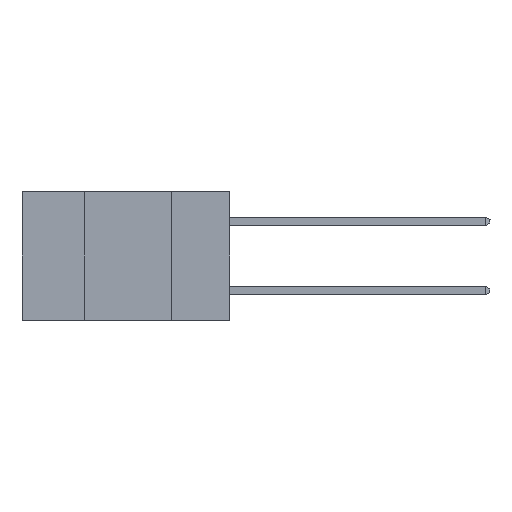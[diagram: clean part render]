
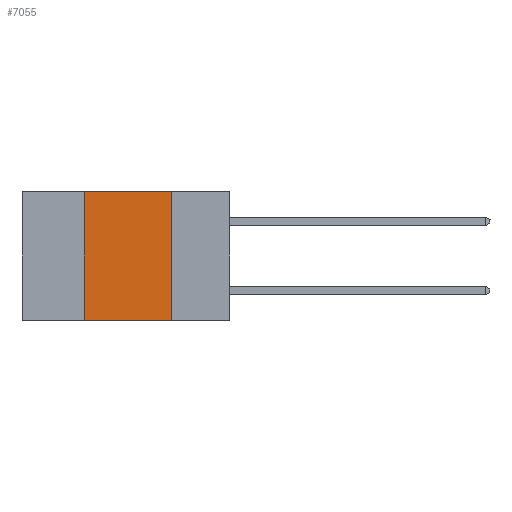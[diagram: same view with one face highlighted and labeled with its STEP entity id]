
A CAD part, left-side view. The second image highlights one B-rep face of the part: STEP entity #7055.
In plain terms, the highlighted planar face has unit normal (-1, 0, 0).
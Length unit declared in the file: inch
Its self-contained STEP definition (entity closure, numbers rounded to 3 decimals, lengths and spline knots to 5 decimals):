
#540 = CARTESIAN_POINT ( 'NONE',  ( 0., 0.6, 0. ) ) ;
#1301 = VECTOR ( 'NONE', #3598, 39.37008 ) ;
#1586 = PLANE ( 'NONE',  #12583 ) ;
#1851 = EDGE_CURVE ( 'NONE', #7175, #4933, #13333, .T. ) ;
#2065 = VECTOR ( 'NONE', #4956, 39.37008 ) ;
#2358 = EDGE_CURVE ( 'NONE', #7175, #4273, #6898, .T. ) ;
#2370 = EDGE_LOOP ( 'NONE', ( #14096, #10110, #2570, #3733 ) ) ;
#2570 = ORIENTED_EDGE ( 'NONE', *, *, #1851, .F. ) ;
#2785 = DIRECTION ( 'NONE',  ( 1., 0., 0. ) ) ;
#3254 = DIRECTION ( 'NONE',  ( 0., 0., 1. ) ) ;
#3525 = CARTESIAN_POINT ( 'NONE',  ( 0., 0.17, -0.37 ) ) ;
#3598 = DIRECTION ( 'NONE',  ( 0., 0., -1. ) ) ;
#3733 = ORIENTED_EDGE ( 'NONE', *, *, #2358, .T. ) ;
#4273 = VERTEX_POINT ( 'NONE', #9576 ) ;
#4481 = VECTOR ( 'NONE', #11503, 39.37008 ) ;
#4933 = VERTEX_POINT ( 'NONE', #9514 ) ;
#4956 = DIRECTION ( 'NONE',  ( 0., -1., 0. ) ) ;
#5850 = FACE_OUTER_BOUND ( 'NONE', #2370, .T. ) ;
#5949 = LINE ( 'NONE', #540, #2065 ) ;
#6898 = LINE ( 'NONE', #12611, #4481 ) ;
#6937 = CARTESIAN_POINT ( 'NONE',  ( 0., 0.17, 0. ) ) ;
#6992 = VERTEX_POINT ( 'NONE', #6937 ) ;
#7055 = ADVANCED_FACE ( 'NONE', ( #5850 ), #1586, .F. ) ;
#7175 = VERTEX_POINT ( 'NONE', #14162 ) ;
#8069 = EDGE_CURVE ( 'NONE', #4933, #6992, #5949, .T. ) ;
#8744 = CARTESIAN_POINT ( 'NONE',  ( 0., 0.42, -0.37 ) ) ;
#9338 = CARTESIAN_POINT ( 'NONE',  ( 0., 0.6, 0. ) ) ;
#9514 = CARTESIAN_POINT ( 'NONE',  ( 0., 0.42, 0. ) ) ;
#9576 = CARTESIAN_POINT ( 'NONE',  ( 0., 0.17, -0.37 ) ) ;
#10110 = ORIENTED_EDGE ( 'NONE', *, *, #8069, .F. ) ;
#10359 = DIRECTION ( 'NONE',  ( 0., 0., -1. ) ) ;
#11503 = DIRECTION ( 'NONE',  ( 0., -1., 0. ) ) ;
#12389 = LINE ( 'NONE', #3525, #1301 ) ;
#12583 = AXIS2_PLACEMENT_3D ( 'NONE', #9338, #2785, #10359 ) ;
#12611 = CARTESIAN_POINT ( 'NONE',  ( 0., 0.6, -0.37 ) ) ;
#13333 = LINE ( 'NONE', #8744, #13723 ) ;
#13723 = VECTOR ( 'NONE', #3254, 39.37008 ) ;
#13889 = EDGE_CURVE ( 'NONE', #6992, #4273, #12389, .T. ) ;
#14096 = ORIENTED_EDGE ( 'NONE', *, *, #13889, .F. ) ;
#14162 = CARTESIAN_POINT ( 'NONE',  ( 0., 0.42, -0.37 ) ) ;
